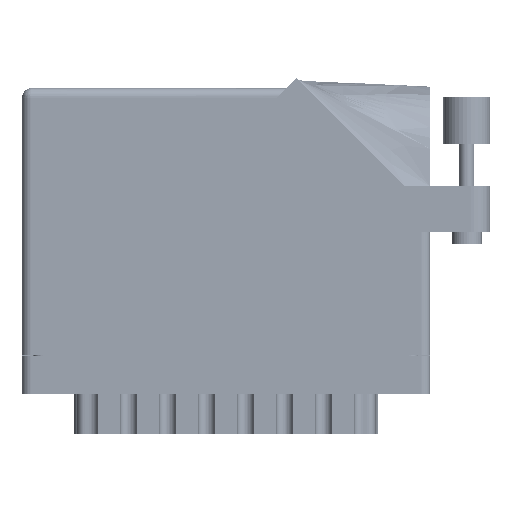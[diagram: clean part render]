
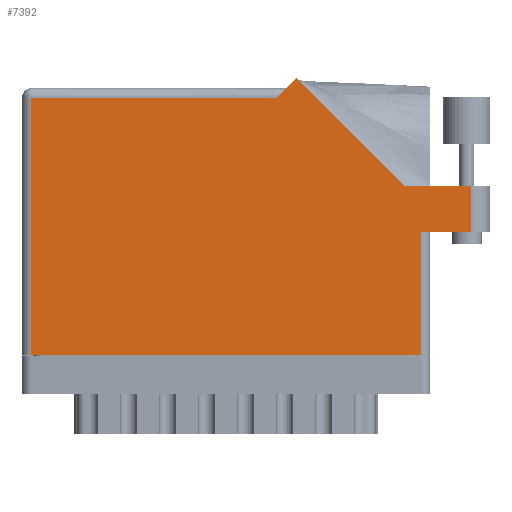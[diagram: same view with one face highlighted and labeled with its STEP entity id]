
A CAD part, front view. The second image highlights one B-rep face of the part: STEP entity #7392.
In plain terms, the highlighted face is planar.
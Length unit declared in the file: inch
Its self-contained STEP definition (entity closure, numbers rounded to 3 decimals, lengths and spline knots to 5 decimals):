
#379 = DIRECTION ( 'NONE',  ( 1., 0., 0. ) ) ;
#1355 = EDGE_CURVE ( 'NONE', #60761, #16707, #55993, .T. ) ;
#4106 = DIRECTION ( 'NONE',  ( 0., 1., 0. ) ) ;
#4125 = EDGE_CURVE ( 'NONE', #16797, #21304, #52965, .T. ) ;
#4636 = CARTESIAN_POINT ( 'NONE',  ( 0., 0., 0. ) ) ;
#7039 = LINE ( 'NONE', #50968, #22979 ) ;
#7167 = VECTOR ( 'NONE', #18310, 39.37008 ) ;
#7392 = ADVANCED_FACE ( 'NONE', ( #35880 ), #33828, .F. ) ;
#7412 = VERTEX_POINT ( 'NONE', #12422 ) ;
#9571 = ORIENTED_EDGE ( 'NONE', *, *, #1355, .T. ) ;
#10556 = DIRECTION ( 'NONE',  ( 1., 0., 0. ) ) ;
#11442 = DIRECTION ( 'NONE',  ( -1., 0., 0. ) ) ;
#12323 = VECTOR ( 'NONE', #55190, 39.37008 ) ;
#12422 = CARTESIAN_POINT ( 'NONE',  ( 2.656, 0., 0. ) ) ;
#12664 = CARTESIAN_POINT ( 'NONE',  ( 3.118, 1.122, 0. ) ) ;
#13760 = VERTEX_POINT ( 'NONE', #29907 ) ;
#14551 = CARTESIAN_POINT ( 'NONE',  ( 1.758, 1.775, 0. ) ) ;
#14561 = LINE ( 'NONE', #4636, #30414 ) ;
#15031 = ORIENTED_EDGE ( 'NONE', *, *, #47051, .T. ) ;
#16403 = CARTESIAN_POINT ( 'NONE',  ( 2.656, 0.815, 0. ) ) ;
#16707 = VERTEX_POINT ( 'NONE', #35946 ) ;
#16797 = VERTEX_POINT ( 'NONE', #47278 ) ;
#17596 = EDGE_CURVE ( 'NONE', #25483, #7412, #14561, .T. ) ;
#18202 = VECTOR ( 'NONE', #379, 39.37008 ) ;
#18310 = DIRECTION ( 'NONE',  ( -1., 0., 0. ) ) ;
#18420 = EDGE_CURVE ( 'NONE', #42700, #16797, #71375, .T. ) ;
#19047 = EDGE_LOOP ( 'NONE', ( #9571, #58872, #55604, #45207, #15031, #69374, #42228, #65570, #67641 ) ) ;
#21304 = VERTEX_POINT ( 'NONE', #40193 ) ;
#21345 = VECTOR ( 'NONE', #56492, 39.37008 ) ;
#22979 = VECTOR ( 'NONE', #45810, 39.37008 ) ;
#25483 = VERTEX_POINT ( 'NONE', #66455 ) ;
#25913 = DIRECTION ( 'NONE',  ( -0.707, -0.707, 0. ) ) ;
#29202 = AXIS2_PLACEMENT_3D ( 'NONE', #33348, #72657, #11442 ) ;
#29907 = CARTESIAN_POINT ( 'NONE',  ( 1.696, 1.713, 0. ) ) ;
#30414 = VECTOR ( 'NONE', #10556, 39.37008 ) ;
#33348 = CARTESIAN_POINT ( 'NONE',  ( 0., 1.775, 0. ) ) ;
#33610 = LINE ( 'NONE', #16403, #54652 ) ;
#33828 = PLANE ( 'NONE',  #29202 ) ;
#35210 = LINE ( 'NONE', #58405, #57224 ) ;
#35880 = FACE_OUTER_BOUND ( 'NONE', #19047, .T. ) ;
#35946 = CARTESIAN_POINT ( 'NONE',  ( 2.993, 0.815, 0. ) ) ;
#37121 = VERTEX_POINT ( 'NONE', #37509 ) ;
#37509 = CARTESIAN_POINT ( 'NONE',  ( 0.062, 1.713, 0. ) ) ;
#38678 = LINE ( 'NONE', #50038, #12323 ) ;
#38727 = EDGE_CURVE ( 'NONE', #37121, #25483, #35210, .T. ) ;
#38976 = EDGE_CURVE ( 'NONE', #16707, #42700, #38678, .T. ) ;
#39468 = LINE ( 'NONE', #14551, #41232 ) ;
#40193 = CARTESIAN_POINT ( 'NONE',  ( 1.82871, 1.84571, 0. ) ) ;
#41232 = VECTOR ( 'NONE', #25913, 39.37008 ) ;
#42228 = ORIENTED_EDGE ( 'NONE', *, *, #38727, .T. ) ;
#42700 = VERTEX_POINT ( 'NONE', #70980 ) ;
#45207 = ORIENTED_EDGE ( 'NONE', *, *, #4125, .T. ) ;
#45810 = DIRECTION ( 'NONE',  ( -1., 0., 0. ) ) ;
#47051 = EDGE_CURVE ( 'NONE', #21304, #13760, #39468, .T. ) ;
#47102 = DIRECTION ( 'NONE',  ( 0., -1., 0. ) ) ;
#47278 = CARTESIAN_POINT ( 'NONE',  ( 2.55242, 1.122, 0. ) ) ;
#50038 = CARTESIAN_POINT ( 'NONE',  ( 2.993, 1.122, 0. ) ) ;
#50968 = CARTESIAN_POINT ( 'NONE',  ( 0., 1.713, 0. ) ) ;
#52965 = LINE ( 'NONE', #56257, #21345 ) ;
#54652 = VECTOR ( 'NONE', #4106, 39.37008 ) ;
#55190 = DIRECTION ( 'NONE',  ( 0., 1., 0. ) ) ;
#55604 = ORIENTED_EDGE ( 'NONE', *, *, #18420, .T. ) ;
#55993 = LINE ( 'NONE', #61677, #18202 ) ;
#56257 = CARTESIAN_POINT ( 'NONE',  ( 2.55242, 1.122, 0. ) ) ;
#56492 = DIRECTION ( 'NONE',  ( -0.707, 0.707, 0. ) ) ;
#57224 = VECTOR ( 'NONE', #47102, 39.37008 ) ;
#58405 = CARTESIAN_POINT ( 'NONE',  ( 0.062, 0., 0. ) ) ;
#58872 = ORIENTED_EDGE ( 'NONE', *, *, #38976, .T. ) ;
#60761 = VERTEX_POINT ( 'NONE', #66480 ) ;
#61677 = CARTESIAN_POINT ( 'NONE',  ( 2.718, 0.815, 0. ) ) ;
#65570 = ORIENTED_EDGE ( 'NONE', *, *, #17596, .T. ) ;
#65922 = EDGE_CURVE ( 'NONE', #7412, #60761, #33610, .T. ) ;
#66455 = CARTESIAN_POINT ( 'NONE',  ( 0.062, 0., 0. ) ) ;
#66480 = CARTESIAN_POINT ( 'NONE',  ( 2.656, 0.815, 0. ) ) ;
#66648 = EDGE_CURVE ( 'NONE', #13760, #37121, #7039, .T. ) ;
#67641 = ORIENTED_EDGE ( 'NONE', *, *, #65922, .T. ) ;
#69374 = ORIENTED_EDGE ( 'NONE', *, *, #66648, .T. ) ;
#70980 = CARTESIAN_POINT ( 'NONE',  ( 2.993, 1.122, 0. ) ) ;
#71375 = LINE ( 'NONE', #12664, #7167 ) ;
#72657 = DIRECTION ( 'NONE',  ( 0., 0., -1. ) ) ;
